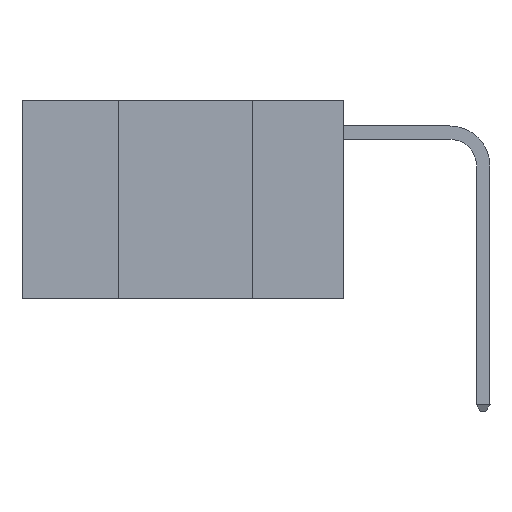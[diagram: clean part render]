
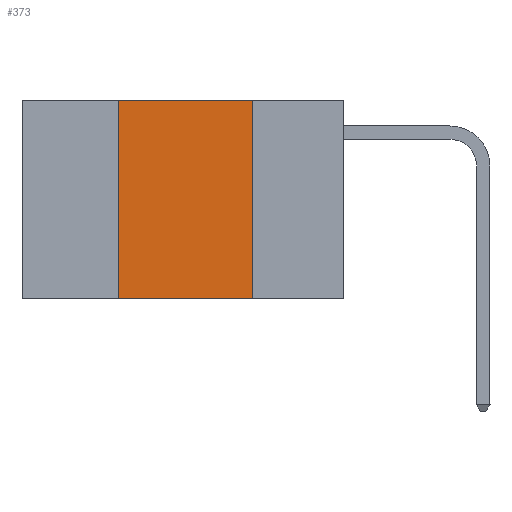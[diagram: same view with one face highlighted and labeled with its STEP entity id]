
A CAD part, left-side view. The second image highlights one B-rep face of the part: STEP entity #373.
In plain terms, the highlighted planar face has unit normal (-1, 0, 0).
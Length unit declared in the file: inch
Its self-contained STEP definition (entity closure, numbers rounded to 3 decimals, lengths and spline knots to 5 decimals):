
#246 = EDGE_LOOP ( 'NONE', ( #14984, #14998, #6043, #13937 ) ) ;
#373 = ADVANCED_FACE ( 'NONE', ( #3785 ), #10903, .F. ) ;
#473 = VERTEX_POINT ( 'NONE', #2656 ) ;
#510 = CARTESIAN_POINT ( 'NONE',  ( 0., 0.17, -0.37 ) ) ;
#1027 = CARTESIAN_POINT ( 'NONE',  ( 0., 0.17, 0. ) ) ;
#1899 = AXIS2_PLACEMENT_3D ( 'NONE', #12289, #5419, #4291 ) ;
#2122 = VERTEX_POINT ( 'NONE', #7340 ) ;
#2293 = VECTOR ( 'NONE', #2519, 39.37008 ) ;
#2519 = DIRECTION ( 'NONE',  ( 0., 0., -1. ) ) ;
#2522 = DIRECTION ( 'NONE',  ( 0., -1., 0. ) ) ;
#2656 = CARTESIAN_POINT ( 'NONE',  ( 0., 0.42, -0.37 ) ) ;
#3785 = FACE_OUTER_BOUND ( 'NONE', #246, .T. ) ;
#4291 = DIRECTION ( 'NONE',  ( 0., 0., -1. ) ) ;
#5034 = LINE ( 'NONE', #8343, #13953 ) ;
#5197 = VECTOR ( 'NONE', #2522, 39.37008 ) ;
#5419 = DIRECTION ( 'NONE',  ( 1., 0., 0. ) ) ;
#5930 = LINE ( 'NONE', #9651, #5197 ) ;
#6043 = ORIENTED_EDGE ( 'NONE', *, *, #11276, .F. ) ;
#7102 = VERTEX_POINT ( 'NONE', #1027 ) ;
#7269 = EDGE_CURVE ( 'NONE', #473, #11460, #13785, .T. ) ;
#7340 = CARTESIAN_POINT ( 'NONE',  ( 0., 0.42, 0. ) ) ;
#7375 = CARTESIAN_POINT ( 'NONE',  ( 0., 0.6, -0.37 ) ) ;
#8343 = CARTESIAN_POINT ( 'NONE',  ( 0., 0.42, 0. ) ) ;
#8591 = DIRECTION ( 'NONE',  ( 0., -1., 0. ) ) ;
#8665 = LINE ( 'NONE', #11975, #2293 ) ;
#9651 = CARTESIAN_POINT ( 'NONE',  ( 0., 0.6, 0. ) ) ;
#10751 = VECTOR ( 'NONE', #8591, 39.37008 ) ;
#10903 = PLANE ( 'NONE',  #1899 ) ;
#11276 = EDGE_CURVE ( 'NONE', #473, #2122, #5034, .T. ) ;
#11460 = VERTEX_POINT ( 'NONE', #510 ) ;
#11843 = DIRECTION ( 'NONE',  ( 0., 0., 1. ) ) ;
#11891 = EDGE_CURVE ( 'NONE', #2122, #7102, #5930, .T. ) ;
#11975 = CARTESIAN_POINT ( 'NONE',  ( 0., 0.17, 0. ) ) ;
#12289 = CARTESIAN_POINT ( 'NONE',  ( 0., 0.6, 0. ) ) ;
#13751 = EDGE_CURVE ( 'NONE', #7102, #11460, #8665, .T. ) ;
#13785 = LINE ( 'NONE', #7375, #10751 ) ;
#13937 = ORIENTED_EDGE ( 'NONE', *, *, #7269, .T. ) ;
#13953 = VECTOR ( 'NONE', #11843, 39.37008 ) ;
#14984 = ORIENTED_EDGE ( 'NONE', *, *, #13751, .F. ) ;
#14998 = ORIENTED_EDGE ( 'NONE', *, *, #11891, .F. ) ;
